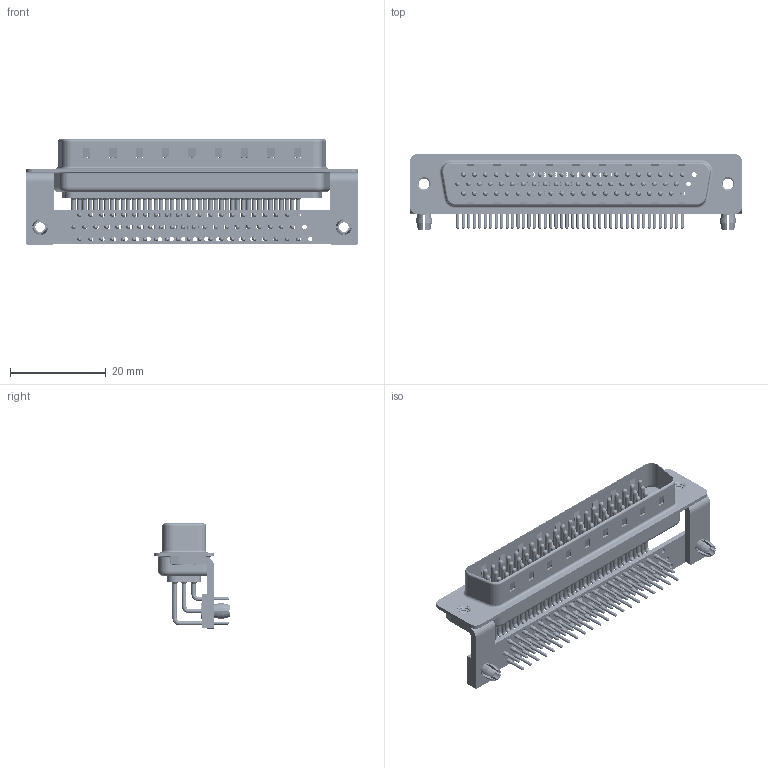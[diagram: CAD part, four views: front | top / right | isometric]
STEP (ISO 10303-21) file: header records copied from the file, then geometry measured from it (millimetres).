
FILE_DESCRIPTION (( 'STEP AP203' ), '1' );
FILE_NAME ('633-M62-663-WN3.STEP', '2018-09-28T04:14:36', ( '' ), ( '' ), 'SwSTEP 2.0', 'SolidWorks 2016', '' );
FILE_SCHEMA (( 'CONFIG_CONTROL_DESIGN' ));
Length unit declared in the file: millimetre
Products named in the file (11): 633M Contact Row 2; 633M Contact Row 3; 633M 4-40 Threaded Rivet_Stabilizer; 633M Stabilizer Bracket; 633M Stabilizer Board_62 Contacts; 633M Housing_62 Contacts; 633M Board Lock; 633M Shell Front_62 Contacts; 633-M62-663-WN3; 633M Shell Rear_62 Contacts; 633M Contact Row 1
Assembly tree (72 placements, depth 2):
  633-M62-663-WN3
    633M Housing_62 Contacts
    633M Shell Front_62 Contacts
    633M Shell Rear_62 Contacts
    633M Contact Row 1  x21
    633M Contact Row 2  x21
    633M Contact Row 3  x20
    633M 4-40 Threaded Rivet_Stabilizer  x2
    633M Stabilizer Bracket  x2
    633M Stabilizer Board_62 Contacts
    633M Board Lock  x2
Bounding box: 69.4 x 15.8 x 22 mm (x, y, z)
Volume: 5119.1 mm3; surface area: 15736.5 mm2
Topology: 72 solids, 72 shells, 7498 faces, 21067 edges, 13728 vertices
Faces by surface type: plane 4245, cylinder 2551, bspline 378, cone 268, torus 56
Entity records: 47694 total; most frequent: CARTESIAN_POINT 9111, DIRECTION 7949, ORIENTED_EDGE 7060, EDGE_CURVE 3530, AXIS2_PLACEMENT_3D 3035, VERTEX_POINT 2310, VECTOR 1879, LINE 1879
